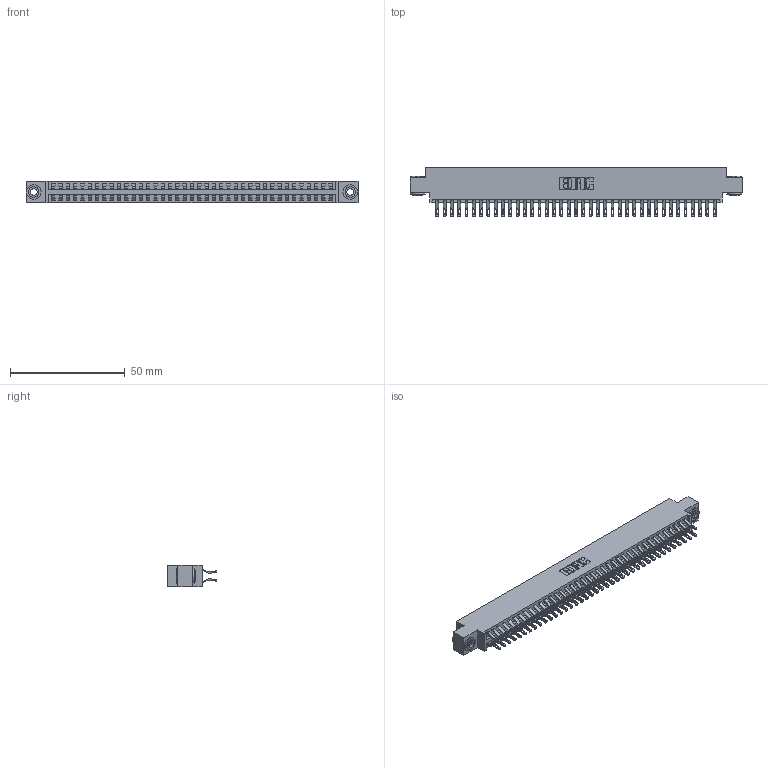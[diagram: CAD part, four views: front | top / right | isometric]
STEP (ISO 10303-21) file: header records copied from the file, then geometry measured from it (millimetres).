
FILE_DESCRIPTION (( 'STEP AP203' ), '1' );
FILE_NAME ('396-078-555-803.STEP', '2019-11-02T13:24:43', ( '' ), ( '' ), 'SwSTEP 2.0', 'SolidWorks 2016', '' );
FILE_SCHEMA (( 'CONFIG_CONTROL_DESIGN' ));
Length unit declared in the file: inch
Products named in the file (4): 345-292-001_555 Tail; 346 Part_0.170 Offset - 0.156 Dia-TH; 345-250-002_345-250-002-102; 396-078-555-803
Assembly tree (81 placements, depth 2):
  396-078-555-803
    346 Part_0.170 Offset - 0.156 Dia-TH
    345-292-001_555 Tail  x78
    345-250-002_345-250-002-102  x2
Bounding box: 144.4 x 21.46 x 9.4 mm (x, y, z)
Volume: 14148.4 mm3; surface area: 20601.1 mm2
Topology: 81 solids, 81 shells, 4688 faces, 14691 edges, 9790 vertices
Faces by surface type: plane 2664, cylinder 2016, cone 8
Entity records: 26964 total; most frequent: CARTESIAN_POINT 4461, ORIENTED_EDGE 4358, DIRECTION 3981, EDGE_CURVE 2179, LINE 1847, VECTOR 1847, VERTEX_POINT 1450, AXIS2_PLACEMENT_3D 1067
